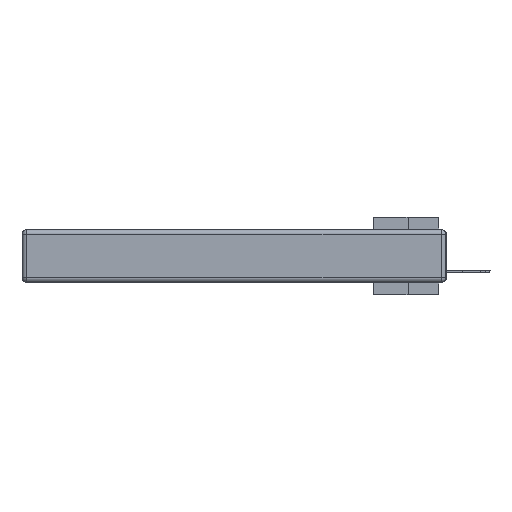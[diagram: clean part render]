
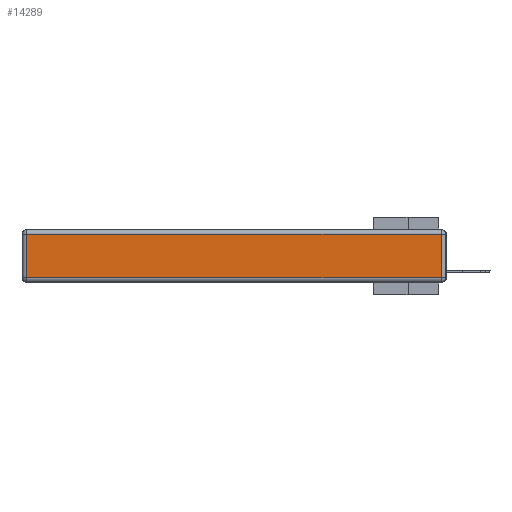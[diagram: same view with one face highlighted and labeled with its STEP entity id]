
A CAD part, left-side view. The second image highlights one B-rep face of the part: STEP entity #14289.
In plain terms, the highlighted planar face has unit normal (-1, 0, 0).
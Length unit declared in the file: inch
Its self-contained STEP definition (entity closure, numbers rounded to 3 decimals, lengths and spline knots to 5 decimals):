
#2321 = EDGE_CURVE ( 'NONE', #27341, #2595, #4677, .T. ) ;
#2595 = VERTEX_POINT ( 'NONE', #5502 ) ;
#3794 = ORIENTED_EDGE ( 'NONE', *, *, #6866, .T. ) ;
#4073 = VECTOR ( 'NONE', #10586, 39.37008 ) ;
#4677 = LINE ( 'NONE', #17572, #19772 ) ;
#5331 = EDGE_CURVE ( 'NONE', #26681, #27341, #27420, .T. ) ;
#5502 = CARTESIAN_POINT ( 'NONE',  ( 0., 0.03, -0.313 ) ) ;
#6866 = EDGE_CURVE ( 'NONE', #2595, #8422, #26241, .T. ) ;
#6901 = EDGE_CURVE ( 'NONE', #8422, #26681, #10005, .T. ) ;
#7125 = ORIENTED_EDGE ( 'NONE', *, *, #6901, .T. ) ;
#7339 = CARTESIAN_POINT ( 'NONE',  ( 0., 2.72, -0.03 ) ) ;
#8422 = VERTEX_POINT ( 'NONE', #11284 ) ;
#9392 = CARTESIAN_POINT ( 'NONE',  ( 0., 2.72, -0.313 ) ) ;
#10005 = LINE ( 'NONE', #19719, #4073 ) ;
#10586 = DIRECTION ( 'NONE',  ( 0., 1., 0. ) ) ;
#10998 = ORIENTED_EDGE ( 'NONE', *, *, #5331, .T. ) ;
#11120 = DIRECTION ( 'NONE',  ( 0., -1., 0. ) ) ;
#11284 = CARTESIAN_POINT ( 'NONE',  ( 0., 0.03, -0.03 ) ) ;
#11891 = VECTOR ( 'NONE', #28376, 39.37008 ) ;
#13763 = EDGE_LOOP ( 'NONE', ( #17083, #3794, #7125, #10998 ) ) ;
#14289 = ADVANCED_FACE ( 'NONE', ( #15460 ), #28369, .T. ) ;
#14778 = DIRECTION ( 'NONE',  ( 0., 0., 1. ) ) ;
#14914 = DIRECTION ( 'NONE',  ( -1., 0., 0. ) ) ;
#15460 = FACE_OUTER_BOUND ( 'NONE', #13763, .T. ) ;
#17083 = ORIENTED_EDGE ( 'NONE', *, *, #2321, .T. ) ;
#17148 = CARTESIAN_POINT ( 'NONE',  ( 0., 0.03, -0.343 ) ) ;
#17572 = CARTESIAN_POINT ( 'NONE',  ( 0., 0., -0.313 ) ) ;
#18715 = AXIS2_PLACEMENT_3D ( 'NONE', #24005, #14914, #26285 ) ;
#19719 = CARTESIAN_POINT ( 'NONE',  ( 0., 2.75, -0.03 ) ) ;
#19772 = VECTOR ( 'NONE', #11120, 39.37008 ) ;
#22716 = VECTOR ( 'NONE', #14778, 39.37008 ) ;
#24005 = CARTESIAN_POINT ( 'NONE',  ( 0., 0., -0.343 ) ) ;
#26241 = LINE ( 'NONE', #17148, #22716 ) ;
#26285 = DIRECTION ( 'NONE',  ( 0., 0., 1. ) ) ;
#26681 = VERTEX_POINT ( 'NONE', #7339 ) ;
#27341 = VERTEX_POINT ( 'NONE', #9392 ) ;
#27420 = LINE ( 'NONE', #28285, #11891 ) ;
#28285 = CARTESIAN_POINT ( 'NONE',  ( 0., 2.72, -0.343 ) ) ;
#28369 = PLANE ( 'NONE',  #18715 ) ;
#28376 = DIRECTION ( 'NONE',  ( 0., 0., -1. ) ) ;
